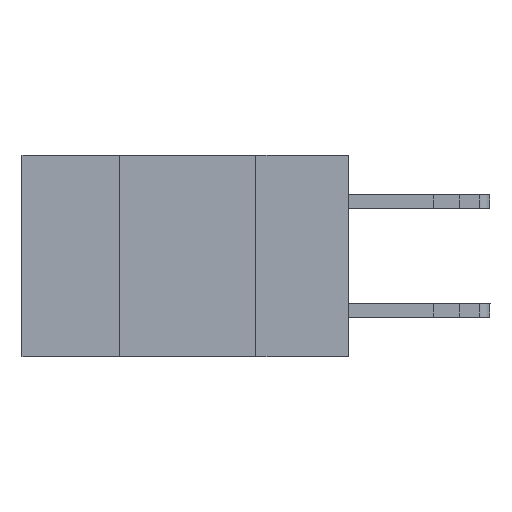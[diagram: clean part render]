
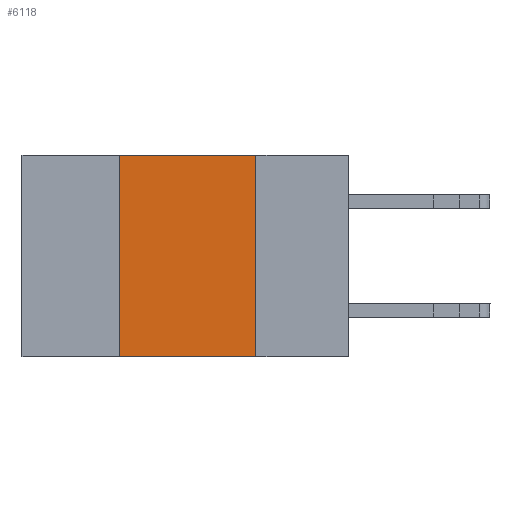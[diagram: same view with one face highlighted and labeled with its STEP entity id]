
A CAD part, left-side view. The second image highlights one B-rep face of the part: STEP entity #6118.
In plain terms, the highlighted planar face has unit normal (-1, 0, 0).
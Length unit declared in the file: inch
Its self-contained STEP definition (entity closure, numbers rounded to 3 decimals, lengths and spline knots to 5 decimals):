
#98 = CARTESIAN_POINT ( 'NONE',  ( 0., 0.42, 0. ) ) ;
#179 = ORIENTED_EDGE ( 'NONE', *, *, #2245, .F. ) ;
#394 = DIRECTION ( 'NONE',  ( 0., 0., -1. ) ) ;
#504 = ORIENTED_EDGE ( 'NONE', *, *, #3172, .F. ) ;
#778 = CARTESIAN_POINT ( 'NONE',  ( 0., 0.6, -0.37 ) ) ;
#1259 = CARTESIAN_POINT ( 'NONE',  ( 0., 0.42, -0.37 ) ) ;
#1971 = FACE_OUTER_BOUND ( 'NONE', #4620, .T. ) ;
#2245 = EDGE_CURVE ( 'NONE', #4397, #5030, #3212, .T. ) ;
#2325 = EDGE_CURVE ( 'NONE', #9710, #4397, #6753, .T. ) ;
#3172 = EDGE_CURVE ( 'NONE', #8447, #9710, #4073, .T. ) ;
#3178 = CARTESIAN_POINT ( 'NONE',  ( 0., 0.17, -0.37 ) ) ;
#3212 = LINE ( 'NONE', #3178, #9613 ) ;
#3305 = CARTESIAN_POINT ( 'NONE',  ( 0., 0.6, 0. ) ) ;
#3366 = PLANE ( 'NONE',  #7715 ) ;
#3741 = EDGE_CURVE ( 'NONE', #8447, #5030, #8562, .T. ) ;
#4073 = LINE ( 'NONE', #1259, #6072 ) ;
#4397 = VERTEX_POINT ( 'NONE', #5210 ) ;
#4620 = EDGE_LOOP ( 'NONE', ( #179, #6245, #504, #6188 ) ) ;
#5030 = VERTEX_POINT ( 'NONE', #6867 ) ;
#5111 = DIRECTION ( 'NONE',  ( 0., 0., 1. ) ) ;
#5210 = CARTESIAN_POINT ( 'NONE',  ( 0., 0.17, 0. ) ) ;
#6000 = DIRECTION ( 'NONE',  ( 0., -1., 0. ) ) ;
#6011 = DIRECTION ( 'NONE',  ( 1., 0., 0. ) ) ;
#6072 = VECTOR ( 'NONE', #5111, 39.37008 ) ;
#6118 = ADVANCED_FACE ( 'NONE', ( #1971 ), #3366, .F. ) ;
#6188 = ORIENTED_EDGE ( 'NONE', *, *, #3741, .T. ) ;
#6245 = ORIENTED_EDGE ( 'NONE', *, *, #2325, .F. ) ;
#6318 = DIRECTION ( 'NONE',  ( 0., -1., 0. ) ) ;
#6647 = DIRECTION ( 'NONE',  ( 0., 0., -1. ) ) ;
#6753 = LINE ( 'NONE', #3305, #10449 ) ;
#6867 = CARTESIAN_POINT ( 'NONE',  ( 0., 0.17, -0.37 ) ) ;
#7715 = AXIS2_PLACEMENT_3D ( 'NONE', #10746, #6011, #394 ) ;
#8289 = VECTOR ( 'NONE', #6318, 39.37008 ) ;
#8447 = VERTEX_POINT ( 'NONE', #11081 ) ;
#8562 = LINE ( 'NONE', #778, #8289 ) ;
#9613 = VECTOR ( 'NONE', #6647, 39.37008 ) ;
#9710 = VERTEX_POINT ( 'NONE', #98 ) ;
#10449 = VECTOR ( 'NONE', #6000, 39.37008 ) ;
#10746 = CARTESIAN_POINT ( 'NONE',  ( 0., 0.6, 0. ) ) ;
#11081 = CARTESIAN_POINT ( 'NONE',  ( 0., 0.42, -0.37 ) ) ;
